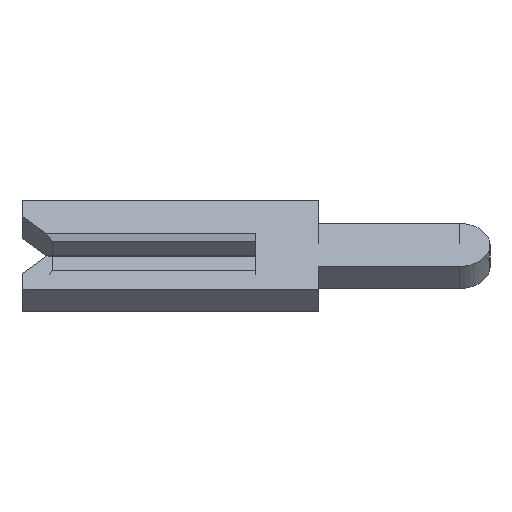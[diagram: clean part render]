
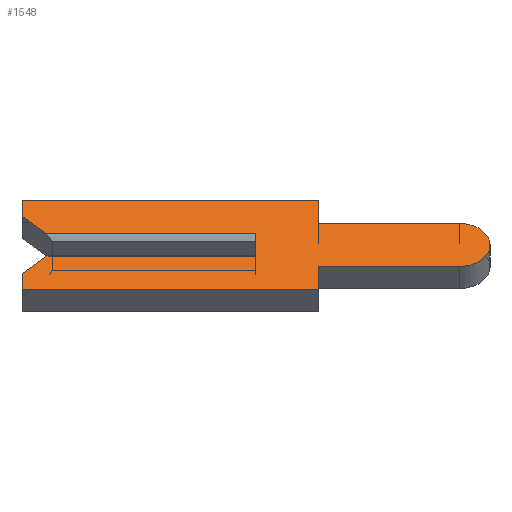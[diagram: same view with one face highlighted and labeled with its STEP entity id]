
A CAD part, left-side view. The second image highlights one B-rep face of the part: STEP entity #1548.
In plain terms, the highlighted face is planar.
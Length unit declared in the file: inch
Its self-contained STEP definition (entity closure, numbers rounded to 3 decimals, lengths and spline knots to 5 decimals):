
#2 = DIRECTION ( 'NONE',  ( 1., 0., 0. ) ) ;
#36 = CARTESIAN_POINT ( 'NONE',  ( -0.01, -0.04, -0.04 ) ) ;
#47 = LINE ( 'NONE', #159, #2419 ) ;
#74 = VERTEX_POINT ( 'NONE', #2551 ) ;
#103 = LINE ( 'NONE', #1628, #1166 ) ;
#158 = EDGE_CURVE ( 'NONE', #2479, #467, #1673, .T. ) ;
#159 = CARTESIAN_POINT ( 'NONE',  ( -0.01, 0.15, 0.04 ) ) ;
#181 = EDGE_LOOP ( 'NONE', ( #2296, #1219, #354, #2220, #492, #453, #1419, #1063, #2829, #950, #778, #257, #707, #1680 ) ) ;
#252 = CARTESIAN_POINT ( 'NONE',  ( -0.01, -0.04, -0.0195 ) ) ;
#257 = ORIENTED_EDGE ( 'NONE', *, *, #1190, .F. ) ;
#261 = CARTESIAN_POINT ( 'NONE',  ( -0.01, -0.1305, -0.01 ) ) ;
#264 = EDGE_CURVE ( 'NONE', #2575, #977, #1567, .T. ) ;
#273 = VECTOR ( 'NONE', #2249, 39.37008 ) ;
#289 = CARTESIAN_POINT ( 'NONE',  ( -0.01, -0.04, 0.0195 ) ) ;
#298 = EDGE_CURVE ( 'NONE', #635, #640, #103, .T. ) ;
#330 = VECTOR ( 'NONE', #1519, 39.37008 ) ;
#335 = LINE ( 'NONE', #2143, #524 ) ;
#354 = ORIENTED_EDGE ( 'NONE', *, *, #2106, .F. ) ;
#361 = EDGE_CURVE ( 'NONE', #640, #526, #1485, .T. ) ;
#369 = DIRECTION ( 'NONE',  ( 0., -1., 0. ) ) ;
#453 = ORIENTED_EDGE ( 'NONE', *, *, #1292, .F. ) ;
#467 = VERTEX_POINT ( 'NONE', #2620 ) ;
#486 = LINE ( 'NONE', #2259, #273 ) ;
#491 = EDGE_CURVE ( 'NONE', #2575, #2825, #2603, .T. ) ;
#492 = ORIENTED_EDGE ( 'NONE', *, *, #2338, .F. ) ;
#506 = CARTESIAN_POINT ( 'NONE',  ( -0.01, 0., 0.01 ) ) ;
#524 = VECTOR ( 'NONE', #2822, 39.37008 ) ;
#526 = VERTEX_POINT ( 'NONE', #2853 ) ;
#635 = VERTEX_POINT ( 'NONE', #2826 ) ;
#640 = VERTEX_POINT ( 'NONE', #1027 ) ;
#660 = VECTOR ( 'NONE', #2782, 39.37008 ) ;
#671 = CARTESIAN_POINT ( 'NONE',  ( -0.01, -0.1305, 0. ) ) ;
#707 = ORIENTED_EDGE ( 'NONE', *, *, #1032, .F. ) ;
#728 = DIRECTION ( 'NONE',  ( 0., -1., 0. ) ) ;
#736 = CARTESIAN_POINT ( 'NONE',  ( -0.01, 0., -0.01 ) ) ;
#778 = ORIENTED_EDGE ( 'NONE', *, *, #298, .F. ) ;
#820 = CARTESIAN_POINT ( 'NONE',  ( -0.01, 0.15, -0.04 ) ) ;
#839 = VECTOR ( 'NONE', #1895, 39.37008 ) ;
#859 = LINE ( 'NONE', #820, #330 ) ;
#887 = LINE ( 'NONE', #261, #1225 ) ;
#917 = CARTESIAN_POINT ( 'NONE',  ( -0.01, -0.1305, 0. ) ) ;
#950 = ORIENTED_EDGE ( 'NONE', *, *, #361, .F. ) ;
#977 = VERTEX_POINT ( 'NONE', #2240 ) ;
#1027 = CARTESIAN_POINT ( 'NONE',  ( -0.01, -0.04, 0.0195 ) ) ;
#1032 = EDGE_CURVE ( 'NONE', #977, #1998, #1337, .T. ) ;
#1036 = DIRECTION ( 'NONE',  ( 0., 0., 1. ) ) ;
#1045 = DIRECTION ( 'NONE',  ( 0., -0.707, 0.707 ) ) ;
#1055 = VECTOR ( 'NONE', #1650, 39.37008 ) ;
#1058 = VERTEX_POINT ( 'NONE', #2003 ) ;
#1063 = ORIENTED_EDGE ( 'NONE', *, *, #2722, .F. ) ;
#1125 = FACE_OUTER_BOUND ( 'NONE', #181, .T. ) ;
#1134 = VECTOR ( 'NONE', #728, 39.37008 ) ;
#1148 = DIRECTION ( 'NONE',  ( 0., 0., 1. ) ) ;
#1166 = VECTOR ( 'NONE', #2344, 39.37008 ) ;
#1172 = DIRECTION ( 'NONE',  ( 0., -1., 0. ) ) ;
#1176 = CARTESIAN_POINT ( 'NONE',  ( -0.01, 0.15, 0.01 ) ) ;
#1184 = CARTESIAN_POINT ( 'NONE',  ( -0.01, 0.134, 0.01 ) ) ;
#1190 = EDGE_CURVE ( 'NONE', #1998, #635, #47, .T. ) ;
#1219 = ORIENTED_EDGE ( 'NONE', *, *, #1697, .F. ) ;
#1225 = VECTOR ( 'NONE', #1172, 39.37008 ) ;
#1292 = EDGE_CURVE ( 'NONE', #467, #1894, #859, .T. ) ;
#1337 = LINE ( 'NONE', #2454, #2092 ) ;
#1414 = CARTESIAN_POINT ( 'NONE',  ( -0.01, 0.1305, 0.0065 ) ) ;
#1419 = ORIENTED_EDGE ( 'NONE', *, *, #158, .F. ) ;
#1485 = LINE ( 'NONE', #289, #1134 ) ;
#1519 = DIRECTION ( 'NONE',  ( 0., 1., 0. ) ) ;
#1548 = ADVANCED_FACE ( 'NONE', ( #1125 ), #2510, .F. ) ;
#1567 = LINE ( 'NONE', #1414, #839 ) ;
#1583 = CARTESIAN_POINT ( 'NONE',  ( -0.01, 0.15, -0.04 ) ) ;
#1604 = EDGE_CURVE ( 'NONE', #74, #2081, #2209, .T. ) ;
#1628 = CARTESIAN_POINT ( 'NONE',  ( -0.01, -0.04, 0.04 ) ) ;
#1635 = CARTESIAN_POINT ( 'NONE',  ( -0.01, 0.15, -0.026 ) ) ;
#1650 = DIRECTION ( 'NONE',  ( 0., 0., -1. ) ) ;
#1673 = LINE ( 'NONE', #36, #1055 ) ;
#1680 = ORIENTED_EDGE ( 'NONE', *, *, #264, .F. ) ;
#1697 = EDGE_CURVE ( 'NONE', #2904, #2825, #486, .T. ) ;
#1793 = DIRECTION ( 'NONE',  ( 1., 0., 0. ) ) ;
#1894 = VERTEX_POINT ( 'NONE', #1583 ) ;
#1895 = DIRECTION ( 'NONE',  ( 0., 0.707, 0.707 ) ) ;
#1998 = VERTEX_POINT ( 'NONE', #2341 ) ;
#2003 = CARTESIAN_POINT ( 'NONE',  ( -0.01, -0.1305, -0.0195 ) ) ;
#2081 = VERTEX_POINT ( 'NONE', #2557 ) ;
#2092 = VECTOR ( 'NONE', #1036, 39.37008 ) ;
#2106 = EDGE_CURVE ( 'NONE', #2081, #2904, #887, .T. ) ;
#2143 = CARTESIAN_POINT ( 'NONE',  ( -0.01, -0.04, -0.0195 ) ) ;
#2209 = LINE ( 'NONE', #2735, #2595 ) ;
#2220 = ORIENTED_EDGE ( 'NONE', *, *, #1604, .F. ) ;
#2240 = CARTESIAN_POINT ( 'NONE',  ( -0.01, 0.15, 0.026 ) ) ;
#2249 = DIRECTION ( 'NONE',  ( 0., 0., 1. ) ) ;
#2259 = CARTESIAN_POINT ( 'NONE',  ( -0.01, 0., 0.0065 ) ) ;
#2269 = DIRECTION ( 'NONE',  ( 0., 0., -1. ) ) ;
#2296 = ORIENTED_EDGE ( 'NONE', *, *, #491, .T. ) ;
#2319 = EDGE_CURVE ( 'NONE', #526, #1058, #2622, .T. ) ;
#2338 = EDGE_CURVE ( 'NONE', #1894, #74, #2809, .T. ) ;
#2341 = CARTESIAN_POINT ( 'NONE',  ( -0.01, 0.15, 0.04 ) ) ;
#2344 = DIRECTION ( 'NONE',  ( 0., 0., -1. ) ) ;
#2419 = VECTOR ( 'NONE', #369, 39.37008 ) ;
#2454 = CARTESIAN_POINT ( 'NONE',  ( -0.01, 0.15, 0.026 ) ) ;
#2479 = VERTEX_POINT ( 'NONE', #252 ) ;
#2510 = PLANE ( 'NONE',  #2703 ) ;
#2537 = DIRECTION ( 'NONE',  ( 0., 0., -1. ) ) ;
#2551 = CARTESIAN_POINT ( 'NONE',  ( -0.01, 0.15, -0.026 ) ) ;
#2557 = CARTESIAN_POINT ( 'NONE',  ( -0.01, 0.134, -0.01 ) ) ;
#2575 = VERTEX_POINT ( 'NONE', #1184 ) ;
#2595 = VECTOR ( 'NONE', #1045, 39.37008 ) ;
#2603 = LINE ( 'NONE', #1176, #660 ) ;
#2620 = CARTESIAN_POINT ( 'NONE',  ( -0.01, -0.04, -0.04 ) ) ;
#2622 = CIRCLE ( 'NONE', #2688, 0.0195 ) ;
#2688 = AXIS2_PLACEMENT_3D ( 'NONE', #917, #2, #2537 ) ;
#2703 = AXIS2_PLACEMENT_3D ( 'NONE', #671, #1793, #2269 ) ;
#2710 = VECTOR ( 'NONE', #1148, 39.37008 ) ;
#2722 = EDGE_CURVE ( 'NONE', #1058, #2479, #335, .T. ) ;
#2735 = CARTESIAN_POINT ( 'NONE',  ( -0.01, 0.1305, -0.0065 ) ) ;
#2782 = DIRECTION ( 'NONE',  ( 0., -1., 0. ) ) ;
#2809 = LINE ( 'NONE', #1635, #2710 ) ;
#2822 = DIRECTION ( 'NONE',  ( 0., 1., 0. ) ) ;
#2825 = VERTEX_POINT ( 'NONE', #506 ) ;
#2826 = CARTESIAN_POINT ( 'NONE',  ( -0.01, -0.04, 0.04 ) ) ;
#2829 = ORIENTED_EDGE ( 'NONE', *, *, #2319, .F. ) ;
#2853 = CARTESIAN_POINT ( 'NONE',  ( -0.01, -0.1305, 0.0195 ) ) ;
#2904 = VERTEX_POINT ( 'NONE', #736 ) ;
